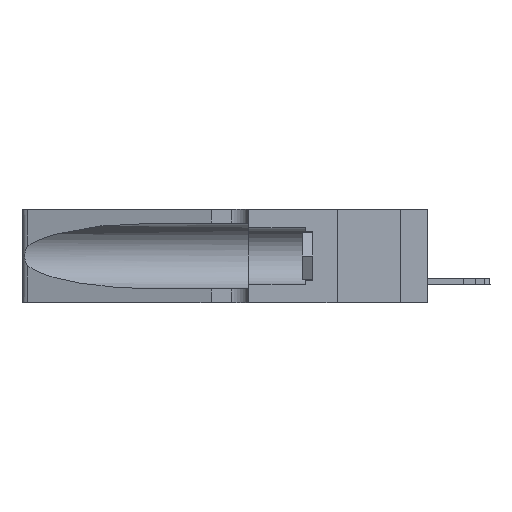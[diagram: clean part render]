
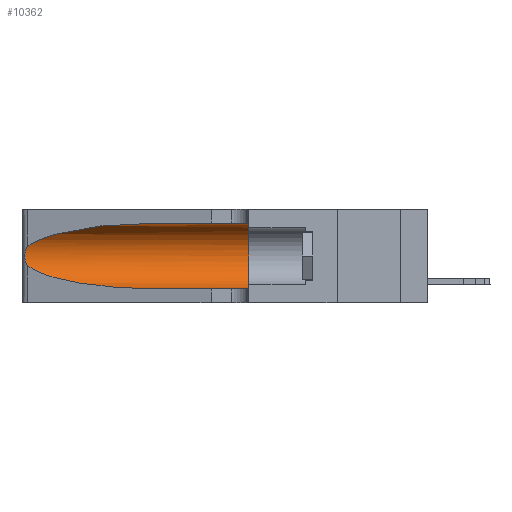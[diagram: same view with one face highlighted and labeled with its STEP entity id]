
A CAD part, left-side view. The second image highlights one B-rep face of the part: STEP entity #10362.
In plain terms, the highlighted cylindrical face has radius 3.308 mm (diameter 6.617 mm), a partial arc.
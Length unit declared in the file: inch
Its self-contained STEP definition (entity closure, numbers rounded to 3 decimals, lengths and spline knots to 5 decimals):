
#39 = EDGE_CURVE ( 'NONE', #625, #4411, #2677, .T. ) ;
#625 = VERTEX_POINT ( 'NONE', #4045 ) ;
#1480 = DIRECTION ( 'NONE',  ( 0., -1., 0. ) ) ;
#2368 = ORIENTED_EDGE ( 'NONE', *, *, #12896, .T. ) ;
#2677 = LINE ( 'NONE', #4526, #17298 ) ;
#3386 = CARTESIAN_POINT ( 'NONE',  ( 0.25854, 1.2359, 0.20912 ) ) ;
#3445 = DIRECTION ( 'NONE',  ( 0., -1., 0. ) ) ;
#4045 = CARTESIAN_POINT ( 'NONE',  ( 0.1305, 0.72297, 0.31525 ) ) ;
#4184 = EDGE_CURVE ( 'NONE', #23387, #8297, #6833, .T. ) ;
#4411 = VERTEX_POINT ( 'NONE', #16897 ) ;
#4526 = CARTESIAN_POINT ( 'NONE',  ( 0.1305, 1.61858, 0.31525 ) ) ;
#5609 = CARTESIAN_POINT ( 'NONE',  ( 0.1305, 0.72297, 0.31525 ) ) ;
#6833 =( BOUNDED_CURVE ( )  B_SPLINE_CURVE ( 3, ( #24075, #12540, #10653, #8709 ),
 .UNSPECIFIED., .F., .F. ) 
 B_SPLINE_CURVE_WITH_KNOTS ( ( 4, 4 ),
 ( 3.44316, 4.71239 ),
 .UNSPECIFIED. ) 
 CURVE ( )  GEOMETRIC_REPRESENTATION_ITEM ( )  RATIONAL_B_SPLINE_CURVE ( ( 1., 0.87, 0.87, 1. ) ) 
 REPRESENTATION_ITEM ( '' )  );
#7163 = CARTESIAN_POINT ( 'NONE',  ( 0.25487, 1.22718, 0.22369 ) ) ;
#7183 = AXIS2_PLACEMENT_3D ( 'NONE', #24373, #10874, #12769 ) ;
#7506 = CARTESIAN_POINT ( 'NONE',  ( 0.25487, 1.22718, 0.22369 ) ) ;
#7797 = FACE_OUTER_BOUND ( 'NONE', #8453, .T. ) ;
#8069 = CARTESIAN_POINT ( 'NONE',  ( 0.1305, 0.72297, 0.05475 ) ) ;
#8297 = VERTEX_POINT ( 'NONE', #8069 ) ;
#8453 = EDGE_LOOP ( 'NONE', ( #20010, #20272, #10059, #2368, #16269, #20660 ) ) ;
#8514 = DIRECTION ( 'NONE',  ( 0., -1., 0. ) ) ;
#8709 = CARTESIAN_POINT ( 'NONE',  ( 0.1305, 0.72297, 0.05475 ) ) ;
#9250 = CARTESIAN_POINT ( 'NONE',  ( 0.18966, 0.96281, 0.31525 ) ) ;
#9262 = CARTESIAN_POINT ( 'NONE',  ( 0.26018, 1.23835, 0.19895 ) ) ;
#9754 = CARTESIAN_POINT ( 'NONE',  ( 0.25789, 1.23486, 0.15765 ) ) ;
#10059 = ORIENTED_EDGE ( 'NONE', *, *, #4184, .T. ) ;
#10362 = ADVANCED_FACE ( 'NONE', ( #7797 ), #10475, .F. ) ;
#10475 = CYLINDRICAL_SURFACE ( 'NONE', #20323, 0.13025 ) ;
#10653 = CARTESIAN_POINT ( 'NONE',  ( 0.18966, 0.96281, 0.05475 ) ) ;
#10874 = DIRECTION ( 'NONE',  ( 0., 1., 0. ) ) ;
#10949 = CIRCLE ( 'NONE', #7183, 0.13025 ) ;
#11163 = CARTESIAN_POINT ( 'NONE',  ( 0.1305, 1.61858, 0.05475 ) ) ;
#11174 = DIRECTION ( 'NONE',  ( 0., 0., -1. ) ) ;
#11385 = CARTESIAN_POINT ( 'NONE',  ( 0.26075, 1.23896, 0.19203 ) ) ;
#11467 = EDGE_CURVE ( 'NONE', #625, #22554, #11605, .T. ) ;
#11605 =( BOUNDED_CURVE ( )  B_SPLINE_CURVE ( 3, ( #5609, #9250, #22865, #22955 ),
 .UNSPECIFIED., .F., .T. ) 
 B_SPLINE_CURVE_WITH_KNOTS ( ( 4, 4 ),
 ( 1.5708, 2.84003 ),
 .UNSPECIFIED. ) 
 CURVE ( )  GEOMETRIC_REPRESENTATION_ITEM ( )  RATIONAL_B_SPLINE_CURVE ( ( 1., 0.87, 0.87, 1. ) ) 
 REPRESENTATION_ITEM ( '' )  );
#12540 = CARTESIAN_POINT ( 'NONE',  ( 0.2373, 1.15595, 0.08982 ) ) ;
#12769 = DIRECTION ( 'NONE',  ( 0., 0., 1. ) ) ;
#12896 = EDGE_CURVE ( 'NONE', #8297, #18829, #18000, .T. ) ;
#13598 = CARTESIAN_POINT ( 'NONE',  ( 0.25856, 1.23593, 0.16098 ) ) ;
#13765 = CARTESIAN_POINT ( 'NONE',  ( 0.25555, 1.22993, 0.14849 ) ) ;
#13841 = EDGE_CURVE ( 'NONE', #22554, #23387, #23046, .T. ) ;
#14047 = CARTESIAN_POINT ( 'NONE',  ( 0.1305, 0.35, 0.05475 ) ) ;
#14998 = CARTESIAN_POINT ( 'NONE',  ( 0.25555, 1.22994, 0.2215 ) ) ;
#15080 = CARTESIAN_POINT ( 'NONE',  ( 0.25787, 1.23484, 0.2124 ) ) ;
#15651 = CARTESIAN_POINT ( 'NONE',  ( 0.25487, 1.22718, 0.14631 ) ) ;
#16269 = ORIENTED_EDGE ( 'NONE', *, *, #19538, .F. ) ;
#16897 = CARTESIAN_POINT ( 'NONE',  ( 0.1305, 0.35, 0.31525 ) ) ;
#17298 = VECTOR ( 'NONE', #8514, 39.37008 ) ;
#17367 = CARTESIAN_POINT ( 'NONE',  ( 0.26017, 1.23833, 0.17102 ) ) ;
#17515 = CARTESIAN_POINT ( 'NONE',  ( 0.25639, 1.23186, 0.15144 ) ) ;
#18000 = LINE ( 'NONE', #11163, #21040 ) ;
#18829 = VERTEX_POINT ( 'NONE', #14047 ) ;
#19229 = CARTESIAN_POINT ( 'NONE',  ( 0.26075, 1.23896, 0.178 ) ) ;
#19367 = CARTESIAN_POINT ( 'NONE',  ( 0.25487, 1.22718, 0.14631 ) ) ;
#19538 = EDGE_CURVE ( 'NONE', #4411, #18829, #10949, .T. ) ;
#20010 = ORIENTED_EDGE ( 'NONE', *, *, #11467, .T. ) ;
#20272 = ORIENTED_EDGE ( 'NONE', *, *, #13841, .T. ) ;
#20323 = AXIS2_PLACEMENT_3D ( 'NONE', #22746, #3445, #11174 ) ;
#20660 = ORIENTED_EDGE ( 'NONE', *, *, #39, .F. ) ;
#21040 = VECTOR ( 'NONE', #1480, 39.37008 ) ;
#22554 = VERTEX_POINT ( 'NONE', #7506 ) ;
#22746 = CARTESIAN_POINT ( 'NONE',  ( 0.1305, 1.61858, 0.185 ) ) ;
#22784 = CARTESIAN_POINT ( 'NONE',  ( 0.25639, 1.23184, 0.21858 ) ) ;
#22865 = CARTESIAN_POINT ( 'NONE',  ( 0.2373, 1.15595, 0.28018 ) ) ;
#22955 = CARTESIAN_POINT ( 'NONE',  ( 0.25487, 1.22718, 0.22369 ) ) ;
#23046 = B_SPLINE_CURVE_WITH_KNOTS ( 'NONE', 3,
 ( #7163, #14998, #22784, #15080, #3386, #9262, #11385, #19229, #17367, #13598, #9754, #17515, #13765, #15651 ),
 .UNSPECIFIED., .F., .F.,
 ( 4, 2, 2, 2, 2, 2, 4 ),
 ( 0., 0.00027, 0.00053, 0.00107, 0.0016, 0.00187, 0.00214 ),
 .UNSPECIFIED. ) ;
#23387 = VERTEX_POINT ( 'NONE', #19367 ) ;
#24075 = CARTESIAN_POINT ( 'NONE',  ( 0.25487, 1.22718, 0.14631 ) ) ;
#24373 = CARTESIAN_POINT ( 'NONE',  ( 0.1305, 0.35, 0.185 ) ) ;
